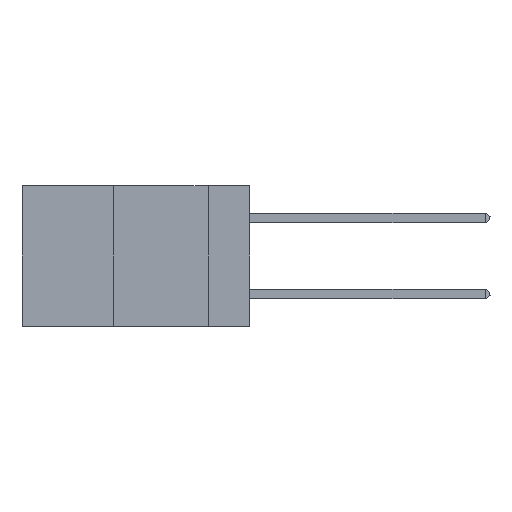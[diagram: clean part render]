
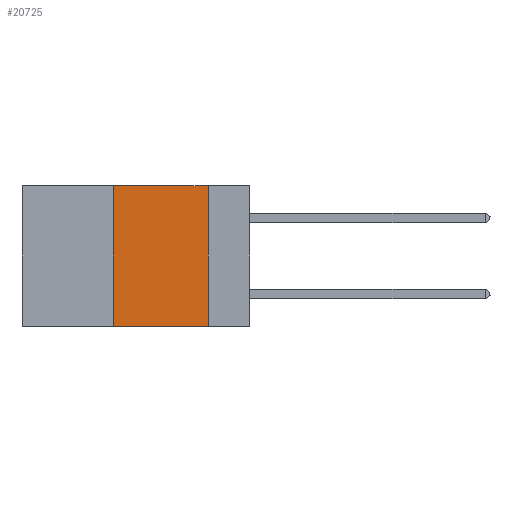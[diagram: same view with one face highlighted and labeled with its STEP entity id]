
A CAD part, left-side view. The second image highlights one B-rep face of the part: STEP entity #20725.
In plain terms, the highlighted planar face has unit normal (-1, 0, 0).
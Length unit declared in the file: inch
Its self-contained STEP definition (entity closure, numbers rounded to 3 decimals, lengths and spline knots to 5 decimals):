
#2446 = VERTEX_POINT ( 'NONE', #2590 ) ;
#2590 = CARTESIAN_POINT ( 'NONE',  ( 0., 0.36, 0. ) ) ;
#3002 = EDGE_CURVE ( 'NONE', #10430, #9929, #12784, .T. ) ;
#5459 = VECTOR ( 'NONE', #29631, 39.37008 ) ;
#8216 = VECTOR ( 'NONE', #37372, 39.37008 ) ;
#8234 = CARTESIAN_POINT ( 'NONE',  ( 0., 0.11, 0. ) ) ;
#9136 = CARTESIAN_POINT ( 'NONE',  ( 0., 0.11, -0.37 ) ) ;
#9929 = VERTEX_POINT ( 'NONE', #9136 ) ;
#10430 = VERTEX_POINT ( 'NONE', #14686 ) ;
#10448 = FACE_OUTER_BOUND ( 'NONE', #12393, .T. ) ;
#10957 = DIRECTION ( 'NONE',  ( 0., 0., -1. ) ) ;
#11277 = LINE ( 'NONE', #13594, #22280 ) ;
#11407 = EDGE_CURVE ( 'NONE', #24485, #9929, #11277, .T. ) ;
#12393 = EDGE_LOOP ( 'NONE', ( #33903, #30914, #19298, #37076 ) ) ;
#12784 = LINE ( 'NONE', #18591, #39601 ) ;
#13116 = PLANE ( 'NONE',  #26782 ) ;
#13594 = CARTESIAN_POINT ( 'NONE',  ( 0., 0.11, 0. ) ) ;
#14085 = CARTESIAN_POINT ( 'NONE',  ( 0., 0.6, 0. ) ) ;
#14686 = CARTESIAN_POINT ( 'NONE',  ( 0., 0.36, -0.37 ) ) ;
#16069 = CARTESIAN_POINT ( 'NONE',  ( 0., 0.6, 0. ) ) ;
#18591 = CARTESIAN_POINT ( 'NONE',  ( 0., 0.6, -0.37 ) ) ;
#18759 = EDGE_CURVE ( 'NONE', #10430, #2446, #20141, .T. ) ;
#19298 = ORIENTED_EDGE ( 'NONE', *, *, #18759, .F. ) ;
#20141 = LINE ( 'NONE', #34166, #8216 ) ;
#20725 = ADVANCED_FACE ( 'NONE', ( #10448 ), #13116, .F. ) ;
#22280 = VECTOR ( 'NONE', #10957, 39.37008 ) ;
#24485 = VERTEX_POINT ( 'NONE', #8234 ) ;
#25540 = LINE ( 'NONE', #14085, #5459 ) ;
#26782 = AXIS2_PLACEMENT_3D ( 'NONE', #16069, #37479, #34674 ) ;
#29631 = DIRECTION ( 'NONE',  ( 0., -1., 0. ) ) ;
#30914 = ORIENTED_EDGE ( 'NONE', *, *, #33511, .F. ) ;
#33511 = EDGE_CURVE ( 'NONE', #2446, #24485, #25540, .T. ) ;
#33903 = ORIENTED_EDGE ( 'NONE', *, *, #11407, .F. ) ;
#34166 = CARTESIAN_POINT ( 'NONE',  ( 0., 0.36, 0. ) ) ;
#34674 = DIRECTION ( 'NONE',  ( 0., 0., -1. ) ) ;
#37076 = ORIENTED_EDGE ( 'NONE', *, *, #3002, .T. ) ;
#37372 = DIRECTION ( 'NONE',  ( 0., 0., 1. ) ) ;
#37479 = DIRECTION ( 'NONE',  ( 1., 0., 0. ) ) ;
#38183 = DIRECTION ( 'NONE',  ( 0., -1., 0. ) ) ;
#39601 = VECTOR ( 'NONE', #38183, 39.37008 ) ;
